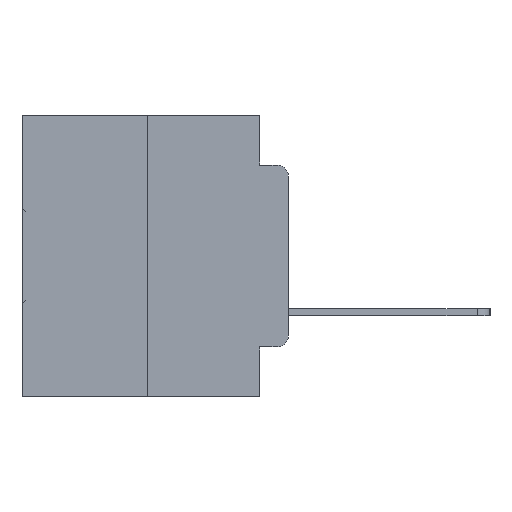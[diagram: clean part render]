
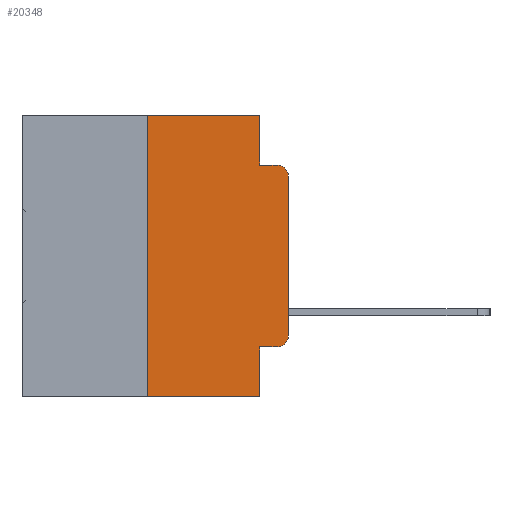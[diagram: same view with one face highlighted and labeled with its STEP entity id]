
A CAD part, left-side view. The second image highlights one B-rep face of the part: STEP entity #20348.
In plain terms, the highlighted planar face has unit normal (-1, 0, 0).
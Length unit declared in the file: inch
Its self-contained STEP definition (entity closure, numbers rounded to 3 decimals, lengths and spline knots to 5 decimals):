
#547 = LINE ( 'NONE', #16850, #12943 ) ;
#661 = DIRECTION ( 'NONE',  ( 0., -1., 0. ) ) ;
#756 = DIRECTION ( 'NONE',  ( 0., 0., 1. ) ) ;
#1582 = CARTESIAN_POINT ( 'NONE',  ( 0., 0.051, -0.0885 ) ) ;
#1742 = ORIENTED_EDGE ( 'NONE', *, *, #10924, .T. ) ;
#1829 = VERTEX_POINT ( 'NONE', #27458 ) ;
#2033 = ORIENTED_EDGE ( 'NONE', *, *, #14547, .F. ) ;
#2270 = CARTESIAN_POINT ( 'NONE',  ( 0., 0.051, 0. ) ) ;
#2423 = CARTESIAN_POINT ( 'NONE',  ( 0., 0.25, 0. ) ) ;
#2908 = FACE_OUTER_BOUND ( 'NONE', #17491, .T. ) ;
#3200 = CARTESIAN_POINT ( 'NONE',  ( 0., 0.051, -0.0885 ) ) ;
#3320 = ORIENTED_EDGE ( 'NONE', *, *, #29550, .T. ) ;
#3491 = EDGE_CURVE ( 'NONE', #5119, #7823, #24886, .T. ) ;
#3605 = CARTESIAN_POINT ( 'NONE',  ( 0., 0.051, -0.4115 ) ) ;
#4129 = DIRECTION ( 'NONE',  ( 0., -1., 0. ) ) ;
#4264 = VERTEX_POINT ( 'NONE', #6616 ) ;
#4716 = EDGE_CURVE ( 'NONE', #1829, #22986, #21473, .T. ) ;
#5119 = VERTEX_POINT ( 'NONE', #26545 ) ;
#5121 = LINE ( 'NONE', #15388, #10854 ) ;
#5648 = VECTOR ( 'NONE', #9449, 39.37008 ) ;
#6020 = CARTESIAN_POINT ( 'NONE',  ( 0., 0.473, 0. ) ) ;
#6616 = CARTESIAN_POINT ( 'NONE',  ( 0., 0.051, -0.5 ) ) ;
#7177 = CARTESIAN_POINT ( 'NONE',  ( 0., 0., -0.1085 ) ) ;
#7335 = DIRECTION ( 'NONE',  ( 0., 0., -1. ) ) ;
#7377 = DIRECTION ( 'NONE',  ( 0., -1., 0. ) ) ;
#7637 = AXIS2_PLACEMENT_3D ( 'NONE', #13472, #30139, #15875 ) ;
#7823 = VERTEX_POINT ( 'NONE', #15091 ) ;
#7903 = VECTOR ( 'NONE', #19331, 39.37008 ) ;
#9433 = ORIENTED_EDGE ( 'NONE', *, *, #18764, .F. ) ;
#9443 = VECTOR ( 'NONE', #756, 39.37008 ) ;
#9449 = DIRECTION ( 'NONE',  ( 0., 0., 1. ) ) ;
#9598 = DIRECTION ( 'NONE',  ( 0., -1., 0. ) ) ;
#10759 = DIRECTION ( 'NONE',  ( -1., 0., 0. ) ) ;
#10854 = VECTOR ( 'NONE', #661, 39.37008 ) ;
#10920 = DIRECTION ( 'NONE',  ( 0., 0., -1. ) ) ;
#10924 = EDGE_CURVE ( 'NONE', #25840, #12706, #5121, .T. ) ;
#11296 = ORIENTED_EDGE ( 'NONE', *, *, #4716, .T. ) ;
#12706 = VERTEX_POINT ( 'NONE', #21402 ) ;
#12796 = VECTOR ( 'NONE', #4129, 39.37008 ) ;
#12943 = VECTOR ( 'NONE', #9598, 39.37008 ) ;
#13056 = CARTESIAN_POINT ( 'NONE',  ( 0., 0.02, -0.0885 ) ) ;
#13472 = CARTESIAN_POINT ( 'NONE',  ( 0., 0.02, -0.1085 ) ) ;
#13545 = LINE ( 'NONE', #1582, #12796 ) ;
#13588 = ORIENTED_EDGE ( 'NONE', *, *, #27715, .T. ) ;
#14547 = EDGE_CURVE ( 'NONE', #29029, #22039, #13545, .T. ) ;
#15068 = LINE ( 'NONE', #2270, #7903 ) ;
#15091 = CARTESIAN_POINT ( 'NONE',  ( 0., 0.25, 0. ) ) ;
#15388 = CARTESIAN_POINT ( 'NONE',  ( 0., 0.051, -0.4115 ) ) ;
#15571 = CARTESIAN_POINT ( 'NONE',  ( 0., 0.051, 0. ) ) ;
#15875 = DIRECTION ( 'NONE',  ( 0., 0., -1. ) ) ;
#16681 = LINE ( 'NONE', #16931, #28616 ) ;
#16850 = CARTESIAN_POINT ( 'NONE',  ( 0., 0.473, 0. ) ) ;
#16931 = CARTESIAN_POINT ( 'NONE',  ( 0., 0.051, 0. ) ) ;
#17343 = ORIENTED_EDGE ( 'NONE', *, *, #20014, .F. ) ;
#17491 = EDGE_LOOP ( 'NONE', ( #11296, #13588, #2033, #9433, #17343, #19980, #18160, #26009, #1742, #3320 ) ) ;
#18160 = ORIENTED_EDGE ( 'NONE', *, *, #29916, .T. ) ;
#18764 = EDGE_CURVE ( 'NONE', #29066, #29029, #16681, .T. ) ;
#19331 = DIRECTION ( 'NONE',  ( 0., 0., -1. ) ) ;
#19389 = CARTESIAN_POINT ( 'NONE',  ( 0., 0.473, -0.5 ) ) ;
#19980 = ORIENTED_EDGE ( 'NONE', *, *, #3491, .F. ) ;
#20014 = EDGE_CURVE ( 'NONE', #7823, #29066, #547, .T. ) ;
#20348 = ADVANCED_FACE ( 'NONE', ( #2908 ), #22898, .F. ) ;
#20909 = LINE ( 'NONE', #19389, #21677 ) ;
#21402 = CARTESIAN_POINT ( 'NONE',  ( 0., 0.02, -0.4115 ) ) ;
#21473 = LINE ( 'NONE', #29741, #9443 ) ;
#21677 = VECTOR ( 'NONE', #7377, 39.37008 ) ;
#22039 = VERTEX_POINT ( 'NONE', #13056 ) ;
#22401 = EDGE_CURVE ( 'NONE', #25840, #4264, #15068, .T. ) ;
#22898 = PLANE ( 'NONE',  #26378 ) ;
#22986 = VERTEX_POINT ( 'NONE', #7177 ) ;
#24059 = CIRCLE ( 'NONE', #7637, 0.02 ) ;
#24886 = LINE ( 'NONE', #2423, #5648 ) ;
#25128 = CARTESIAN_POINT ( 'NONE',  ( 0., 0.02, -0.3915 ) ) ;
#25285 = DIRECTION ( 'NONE',  ( 1., 0., 0. ) ) ;
#25840 = VERTEX_POINT ( 'NONE', #3605 ) ;
#26009 = ORIENTED_EDGE ( 'NONE', *, *, #22401, .F. ) ;
#26378 = AXIS2_PLACEMENT_3D ( 'NONE', #6020, #25285, #10920 ) ;
#26545 = CARTESIAN_POINT ( 'NONE',  ( 0., 0.25, -0.5 ) ) ;
#27458 = CARTESIAN_POINT ( 'NONE',  ( 0., 0., -0.3915 ) ) ;
#27512 = DIRECTION ( 'NONE',  ( 0., 0., -1. ) ) ;
#27715 = EDGE_CURVE ( 'NONE', #22986, #22039, #24059, .T. ) ;
#28616 = VECTOR ( 'NONE', #7335, 39.37008 ) ;
#28728 = AXIS2_PLACEMENT_3D ( 'NONE', #25128, #10759, #27512 ) ;
#29029 = VERTEX_POINT ( 'NONE', #3200 ) ;
#29066 = VERTEX_POINT ( 'NONE', #15571 ) ;
#29550 = EDGE_CURVE ( 'NONE', #12706, #1829, #31316, .T. ) ;
#29741 = CARTESIAN_POINT ( 'NONE',  ( 0., 0., 0. ) ) ;
#29916 = EDGE_CURVE ( 'NONE', #5119, #4264, #20909, .T. ) ;
#30139 = DIRECTION ( 'NONE',  ( -1., 0., 0. ) ) ;
#31316 = CIRCLE ( 'NONE', #28728, 0.02 ) ;
